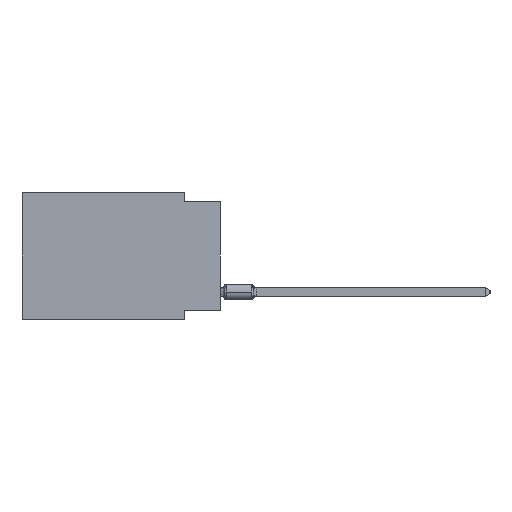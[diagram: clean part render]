
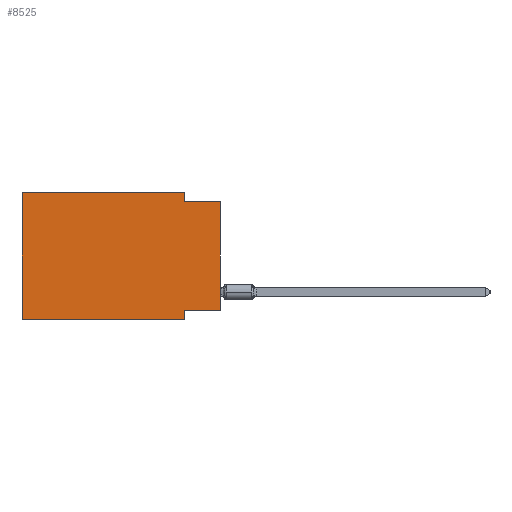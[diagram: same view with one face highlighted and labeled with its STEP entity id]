
A CAD part, left-side view. The second image highlights one B-rep face of the part: STEP entity #8525.
In plain terms, the highlighted planar face has unit normal (-1, 0, 0).
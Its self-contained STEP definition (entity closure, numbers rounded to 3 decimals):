
#667 = CARTESIAN_POINT ( 'NONE',  ( 0., 0., 0. ) ) ;
#1128 = DIRECTION ( 'NONE',  ( 0., 0., 1. ) ) ;
#1442 = VECTOR ( 'NONE', #40601, 1000. ) ;
#1481 = LINE ( 'NONE', #19162, #15433 ) ;
#1483 = CARTESIAN_POINT ( 'NONE',  ( 0., 2.54, -0.635 ) ) ;
#1846 = ORIENTED_EDGE ( 'NONE', *, *, #34416, .F. ) ;
#1861 = CARTESIAN_POINT ( 'NONE',  ( 0., 2.54, 0. ) ) ;
#1888 = FACE_OUTER_BOUND ( 'NONE', #44639, .T. ) ;
#2353 = AXIS2_PLACEMENT_3D ( 'NONE', #5400, #13232, #16744 ) ;
#2721 = VERTEX_POINT ( 'NONE', #1483 ) ;
#3643 = ORIENTED_EDGE ( 'NONE', *, *, #4898, .T. ) ;
#4107 = CARTESIAN_POINT ( 'NONE',  ( 0., 13.97, 0. ) ) ;
#4321 = LINE ( 'NONE', #4107, #4831 ) ;
#4831 = VECTOR ( 'NONE', #35868, 1000. ) ;
#4898 = EDGE_CURVE ( 'NONE', #37190, #33392, #23209, .T. ) ;
#5400 = CARTESIAN_POINT ( 'NONE',  ( 0., 13.97, 0. ) ) ;
#5841 = VECTOR ( 'NONE', #12860, 1000. ) ;
#6477 = LINE ( 'NONE', #1861, #14629 ) ;
#6573 = LINE ( 'NONE', #31390, #5841 ) ;
#6682 = EDGE_CURVE ( 'NONE', #37686, #31470, #18575, .T. ) ;
#7028 = ORIENTED_EDGE ( 'NONE', *, *, #34054, .F. ) ;
#8067 = VECTOR ( 'NONE', #9662, 1000. ) ;
#8525 = ADVANCED_FACE ( 'NONE', ( #1888 ), #16056, .F. ) ;
#9355 = ORIENTED_EDGE ( 'NONE', *, *, #17469, .F. ) ;
#9662 = DIRECTION ( 'NONE',  ( 0., 0., -1. ) ) ;
#12860 = DIRECTION ( 'NONE',  ( 0., -1., 0. ) ) ;
#13232 = DIRECTION ( 'NONE',  ( 1., 0., 0. ) ) ;
#13854 = VERTEX_POINT ( 'NONE', #14605 ) ;
#14605 = CARTESIAN_POINT ( 'NONE',  ( 0., 2.54, -8.255 ) ) ;
#14629 = VECTOR ( 'NONE', #19761, 1000. ) ;
#15433 = VECTOR ( 'NONE', #18462, 1000. ) ;
#16056 = PLANE ( 'NONE',  #2353 ) ;
#16119 = VERTEX_POINT ( 'NONE', #32235 ) ;
#16744 = DIRECTION ( 'NONE',  ( 0., 0., -1. ) ) ;
#17469 = EDGE_CURVE ( 'NONE', #18647, #16119, #4321, .T. ) ;
#18462 = DIRECTION ( 'NONE',  ( 0., 1., 0. ) ) ;
#18575 = LINE ( 'NONE', #667, #37771 ) ;
#18647 = VERTEX_POINT ( 'NONE', #25077 ) ;
#19162 = CARTESIAN_POINT ( 'NONE',  ( 0., 0., -8.255 ) ) ;
#19761 = DIRECTION ( 'NONE',  ( 0., 0., -1. ) ) ;
#22711 = CARTESIAN_POINT ( 'NONE',  ( 0., 0., -8.255 ) ) ;
#23209 = LINE ( 'NONE', #30368, #1442 ) ;
#25077 = CARTESIAN_POINT ( 'NONE',  ( 0., 13.97, 0. ) ) ;
#28071 = EDGE_CURVE ( 'NONE', #16119, #2721, #6477, .T. ) ;
#29465 = ORIENTED_EDGE ( 'NONE', *, *, #28071, .F. ) ;
#30368 = CARTESIAN_POINT ( 'NONE',  ( 0., 13.97, -8.89 ) ) ;
#31390 = CARTESIAN_POINT ( 'NONE',  ( 0., 0., -0.635 ) ) ;
#31470 = VERTEX_POINT ( 'NONE', #42431 ) ;
#31550 = LINE ( 'NONE', #45730, #41643 ) ;
#32235 = CARTESIAN_POINT ( 'NONE',  ( 0., 2.54, 0. ) ) ;
#33392 = VERTEX_POINT ( 'NONE', #40318 ) ;
#34054 = EDGE_CURVE ( 'NONE', #13854, #33392, #41429, .T. ) ;
#34416 = EDGE_CURVE ( 'NONE', #2721, #31470, #6573, .T. ) ;
#35720 = ORIENTED_EDGE ( 'NONE', *, *, #6682, .T. ) ;
#35868 = DIRECTION ( 'NONE',  ( 0., -1., 0. ) ) ;
#37190 = VERTEX_POINT ( 'NONE', #42633 ) ;
#37478 = ORIENTED_EDGE ( 'NONE', *, *, #40280, .F. ) ;
#37686 = VERTEX_POINT ( 'NONE', #22711 ) ;
#37771 = VECTOR ( 'NONE', #1128, 1000. ) ;
#38176 = CARTESIAN_POINT ( 'NONE',  ( 0., 2.54, -8.89 ) ) ;
#39143 = ORIENTED_EDGE ( 'NONE', *, *, #41802, .F. ) ;
#40280 = EDGE_CURVE ( 'NONE', #37190, #18647, #31550, .T. ) ;
#40318 = CARTESIAN_POINT ( 'NONE',  ( 0., 2.54, -8.89 ) ) ;
#40601 = DIRECTION ( 'NONE',  ( 0., -1., 0. ) ) ;
#41429 = LINE ( 'NONE', #38176, #8067 ) ;
#41643 = VECTOR ( 'NONE', #42227, 1000. ) ;
#41802 = EDGE_CURVE ( 'NONE', #37686, #13854, #1481, .T. ) ;
#42227 = DIRECTION ( 'NONE',  ( 0., 0., 1. ) ) ;
#42431 = CARTESIAN_POINT ( 'NONE',  ( 0., 0., -0.635 ) ) ;
#42633 = CARTESIAN_POINT ( 'NONE',  ( 0., 13.97, -8.89 ) ) ;
#44639 = EDGE_LOOP ( 'NONE', ( #35720, #1846, #29465, #9355, #37478, #3643, #7028, #39143 ) ) ;
#45730 = CARTESIAN_POINT ( 'NONE',  ( 0., 13.97, 0. ) ) ;
